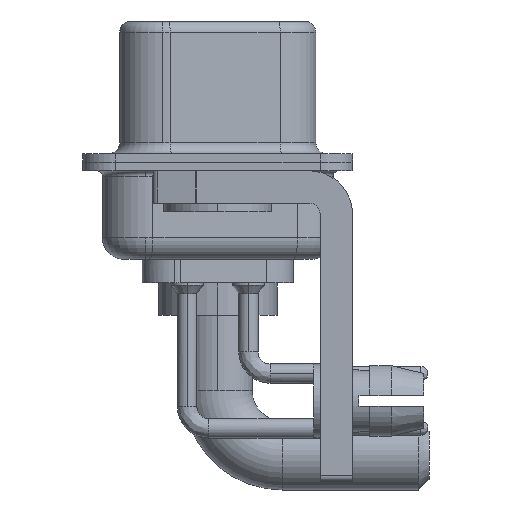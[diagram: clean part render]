
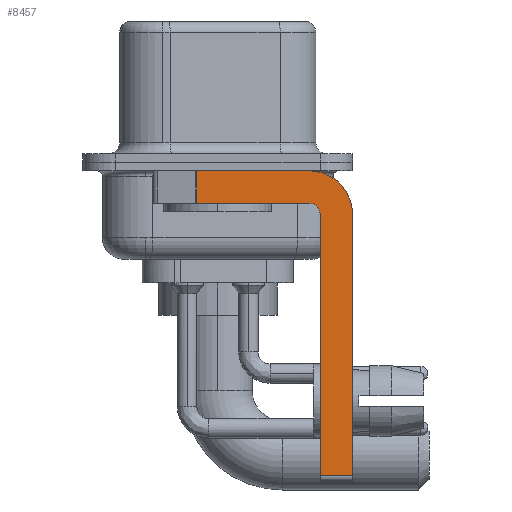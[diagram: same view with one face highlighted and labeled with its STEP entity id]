
A CAD part, left-side view. The second image highlights one B-rep face of the part: STEP entity #8457.
In plain terms, the highlighted planar face has unit normal (-1, 0, 0).
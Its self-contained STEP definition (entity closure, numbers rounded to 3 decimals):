
#400 = VERTEX_POINT ( 'NONE', #13644 ) ;
#596 = ORIENTED_EDGE ( 'NONE', *, *, #10254, .F. ) ;
#731 = DIRECTION ( 'NONE',  ( 0., -1., 0. ) ) ;
#1045 = CARTESIAN_POINT ( 'NONE',  ( -2.9, -4.25, -2.4 ) ) ;
#1092 = DIRECTION ( 'NONE',  ( 0., -1., 0. ) ) ;
#1163 = CIRCLE ( 'NONE', #2219, 2. ) ;
#1178 = DIRECTION ( 'NONE',  ( 0., 0., -1. ) ) ;
#1399 = LINE ( 'NONE', #11090, #6292 ) ;
#1876 = EDGE_CURVE ( 'NONE', #6667, #13525, #12691, .T. ) ;
#2219 = AXIS2_PLACEMENT_3D ( 'NONE', #2614, #4692, #19427 ) ;
#2614 = CARTESIAN_POINT ( 'NONE',  ( -2.9, -4.25, -2.4 ) ) ;
#2714 = ORIENTED_EDGE ( 'NONE', *, *, #6836, .F. ) ;
#2921 = ORIENTED_EDGE ( 'NONE', *, *, #8530, .F. ) ;
#4070 = DIRECTION ( 'NONE',  ( 0., 0., -1. ) ) ;
#4092 = VECTOR ( 'NONE', #731, 1000. ) ;
#4511 = DIRECTION ( 'NONE',  ( 0., 0., -1. ) ) ;
#4674 = AXIS2_PLACEMENT_3D ( 'NONE', #17884, #7992, #1178 ) ;
#4692 = DIRECTION ( 'NONE',  ( 1., 0., 0. ) ) ;
#4819 = EDGE_CURVE ( 'NONE', #400, #20889, #19574, .T. ) ;
#4926 = ORIENTED_EDGE ( 'NONE', *, *, #13007, .F. ) ;
#5113 = VECTOR ( 'NONE', #13577, 1000. ) ;
#5436 = CIRCLE ( 'NONE', #11397, 0.5 ) ;
#5695 = LINE ( 'NONE', #10745, #15627 ) ;
#5697 = CARTESIAN_POINT ( 'NONE',  ( -2.9, -6.25, -2.4 ) ) ;
#5928 = LINE ( 'NONE', #20772, #13641 ) ;
#6216 = EDGE_CURVE ( 'NONE', #400, #10874, #1399, .T. ) ;
#6292 = VECTOR ( 'NONE', #1092, 1000. ) ;
#6639 = VECTOR ( 'NONE', #4511, 1000. ) ;
#6667 = VERTEX_POINT ( 'NONE', #21185 ) ;
#6729 = VERTEX_POINT ( 'NONE', #9522 ) ;
#6836 = EDGE_CURVE ( 'NONE', #6729, #20889, #16885, .T. ) ;
#7508 = CARTESIAN_POINT ( 'NONE',  ( -2.9, -4.25, -0.4 ) ) ;
#7574 = EDGE_LOOP ( 'NONE', ( #9097, #10246, #2714, #596, #9868, #8536, #4926, #2921 ) ) ;
#7933 = CARTESIAN_POINT ( 'NONE',  ( -2.9, -4.75, -2.4 ) ) ;
#7956 = VERTEX_POINT ( 'NONE', #5697 ) ;
#7992 = DIRECTION ( 'NONE',  ( 1., 0., 0. ) ) ;
#8457 = ADVANCED_FACE ( 'NONE', ( #9200 ), #14363, .F. ) ;
#8530 = EDGE_CURVE ( 'NONE', #10874, #7956, #1163, .T. ) ;
#8536 = ORIENTED_EDGE ( 'NONE', *, *, #1876, .T. ) ;
#9097 = ORIENTED_EDGE ( 'NONE', *, *, #6216, .F. ) ;
#9200 = FACE_OUTER_BOUND ( 'NONE', #7574, .T. ) ;
#9283 = DIRECTION ( 'NONE',  ( 0., 0., 1. ) ) ;
#9522 = CARTESIAN_POINT ( 'NONE',  ( -2.9, -4.25, -1.9 ) ) ;
#9868 = ORIENTED_EDGE ( 'NONE', *, *, #20811, .F. ) ;
#10246 = ORIENTED_EDGE ( 'NONE', *, *, #4819, .T. ) ;
#10254 = EDGE_CURVE ( 'NONE', #19598, #6729, #5436, .T. ) ;
#10525 = CARTESIAN_POINT ( 'NONE',  ( -2.9, 0.978, -1.9 ) ) ;
#10638 = DIRECTION ( 'NONE',  ( 0., 0., 1. ) ) ;
#10745 = CARTESIAN_POINT ( 'NONE',  ( -2.9, -4.75, -14.8 ) ) ;
#10874 = VERTEX_POINT ( 'NONE', #7508 ) ;
#11090 = CARTESIAN_POINT ( 'NONE',  ( -2.9, 3., -0.4 ) ) ;
#11397 = AXIS2_PLACEMENT_3D ( 'NONE', #1045, #19515, #9283 ) ;
#12691 = LINE ( 'NONE', #14455, #4092 ) ;
#13007 = EDGE_CURVE ( 'NONE', #7956, #13525, #5928, .T. ) ;
#13525 = VERTEX_POINT ( 'NONE', #16643 ) ;
#13577 = DIRECTION ( 'NONE',  ( 0., 1., 0. ) ) ;
#13641 = VECTOR ( 'NONE', #4070, 1000. ) ;
#13644 = CARTESIAN_POINT ( 'NONE',  ( -2.9, 0.978, -0.4 ) ) ;
#14183 = CARTESIAN_POINT ( 'NONE',  ( -2.9, 0.978, -1.9 ) ) ;
#14363 = PLANE ( 'NONE',  #4674 ) ;
#14455 = CARTESIAN_POINT ( 'NONE',  ( -2.9, -4.25, -14.55 ) ) ;
#15119 = CARTESIAN_POINT ( 'NONE',  ( -2.9, -4.25, -1.9 ) ) ;
#15627 = VECTOR ( 'NONE', #10638, 1000. ) ;
#16643 = CARTESIAN_POINT ( 'NONE',  ( -2.9, -6.25, -14.55 ) ) ;
#16885 = LINE ( 'NONE', #15119, #5113 ) ;
#17884 = CARTESIAN_POINT ( 'NONE',  ( -2.9, -4.25, -2.4 ) ) ;
#19427 = DIRECTION ( 'NONE',  ( 0., 0., -1. ) ) ;
#19515 = DIRECTION ( 'NONE',  ( -1., 0., 0. ) ) ;
#19574 = LINE ( 'NONE', #14183, #6639 ) ;
#19598 = VERTEX_POINT ( 'NONE', #7933 ) ;
#20772 = CARTESIAN_POINT ( 'NONE',  ( -2.9, -6.25, -2.4 ) ) ;
#20811 = EDGE_CURVE ( 'NONE', #6667, #19598, #5695, .T. ) ;
#20889 = VERTEX_POINT ( 'NONE', #10525 ) ;
#21185 = CARTESIAN_POINT ( 'NONE',  ( -2.9, -4.75, -14.55 ) ) ;
